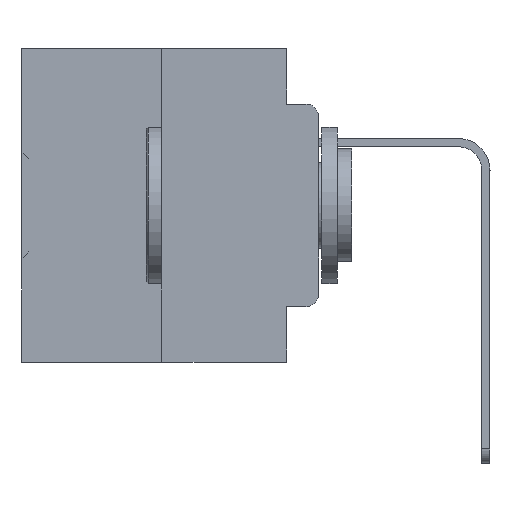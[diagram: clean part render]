
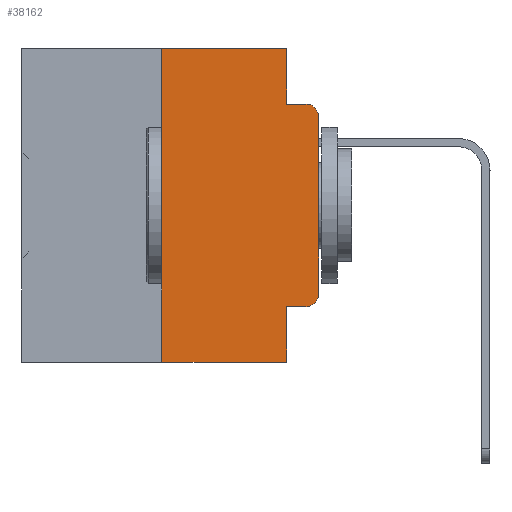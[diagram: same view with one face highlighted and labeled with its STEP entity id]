
A CAD part, left-side view. The second image highlights one B-rep face of the part: STEP entity #38162.
In plain terms, the highlighted planar face has unit normal (-1, 0, 0).
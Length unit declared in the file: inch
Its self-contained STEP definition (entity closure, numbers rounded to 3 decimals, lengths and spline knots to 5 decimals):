
#344 = DIRECTION ( 'NONE',  ( 0., -1., 0. ) ) ;
#496 = CARTESIAN_POINT ( 'NONE',  ( 0., 0.25, -0.5 ) ) ;
#507 = VECTOR ( 'NONE', #17823, 39.37008 ) ;
#673 = CARTESIAN_POINT ( 'NONE',  ( 0., 0.051, 0. ) ) ;
#3181 = VERTEX_POINT ( 'NONE', #29579 ) ;
#3183 = VERTEX_POINT ( 'NONE', #11912 ) ;
#3222 = CARTESIAN_POINT ( 'NONE',  ( 0., 0.473, -0.5 ) ) ;
#3623 = VERTEX_POINT ( 'NONE', #23403 ) ;
#4198 = ORIENTED_EDGE ( 'NONE', *, *, #27834, .T. ) ;
#4359 = LINE ( 'NONE', #6867, #10479 ) ;
#4739 = CARTESIAN_POINT ( 'NONE',  ( 0., 0.25, 0. ) ) ;
#5105 = ORIENTED_EDGE ( 'NONE', *, *, #22924, .T. ) ;
#5196 = FACE_OUTER_BOUND ( 'NONE', #33739, .T. ) ;
#6677 = AXIS2_PLACEMENT_3D ( 'NONE', #27060, #35985, #32703 ) ;
#6692 = EDGE_CURVE ( 'NONE', #25828, #33305, #9351, .T. ) ;
#6867 = CARTESIAN_POINT ( 'NONE',  ( 0., 0.473, 0. ) ) ;
#7886 = ORIENTED_EDGE ( 'NONE', *, *, #18816, .F. ) ;
#8548 = VECTOR ( 'NONE', #34842, 39.37008 ) ;
#9351 = LINE ( 'NONE', #18207, #34954 ) ;
#10479 = VECTOR ( 'NONE', #18948, 39.37008 ) ;
#10750 = EDGE_CURVE ( 'NONE', #22119, #18184, #4359, .T. ) ;
#11199 = ORIENTED_EDGE ( 'NONE', *, *, #17711, .F. ) ;
#11912 = CARTESIAN_POINT ( 'NONE',  ( 0., 0.051, -0.5 ) ) ;
#12039 = AXIS2_PLACEMENT_3D ( 'NONE', #25235, #18634, #13546 ) ;
#13354 = EDGE_CURVE ( 'NONE', #18184, #19110, #32192, .T. ) ;
#13495 = DIRECTION ( 'NONE',  ( 0., -1., 0. ) ) ;
#13541 = CARTESIAN_POINT ( 'NONE',  ( 0., 0.02, -0.3915 ) ) ;
#13546 = DIRECTION ( 'NONE',  ( 0., 0., -1. ) ) ;
#16390 = VECTOR ( 'NONE', #13495, 39.37008 ) ;
#17711 = EDGE_CURVE ( 'NONE', #35717, #22119, #23434, .T. ) ;
#17823 = DIRECTION ( 'NONE',  ( 0., -1., 0. ) ) ;
#18184 = VERTEX_POINT ( 'NONE', #673 ) ;
#18207 = CARTESIAN_POINT ( 'NONE',  ( 0., 0.051, -0.4115 ) ) ;
#18286 = LINE ( 'NONE', #34178, #16390 ) ;
#18634 = DIRECTION ( 'NONE',  ( -1., 0., 0. ) ) ;
#18816 = EDGE_CURVE ( 'NONE', #19110, #3181, #18286, .T. ) ;
#18948 = DIRECTION ( 'NONE',  ( 0., -1., 0. ) ) ;
#19110 = VERTEX_POINT ( 'NONE', #22458 ) ;
#19937 = ORIENTED_EDGE ( 'NONE', *, *, #6692, .T. ) ;
#20440 = LINE ( 'NONE', #25420, #37202 ) ;
#21006 = EDGE_CURVE ( 'NONE', #25828, #3183, #20440, .T. ) ;
#21831 = CARTESIAN_POINT ( 'NONE',  ( 0., 0.051, -0.4115 ) ) ;
#22119 = VERTEX_POINT ( 'NONE', #35613 ) ;
#22409 = ORIENTED_EDGE ( 'NONE', *, *, #34495, .T. ) ;
#22458 = CARTESIAN_POINT ( 'NONE',  ( 0., 0.051, -0.0885 ) ) ;
#22924 = EDGE_CURVE ( 'NONE', #35196, #3181, #33763, .T. ) ;
#23353 = VECTOR ( 'NONE', #23436, 39.37008 ) ;
#23403 = CARTESIAN_POINT ( 'NONE',  ( 0., 0., -0.3915 ) ) ;
#23434 = LINE ( 'NONE', #4739, #8548 ) ;
#23436 = DIRECTION ( 'NONE',  ( 0., 0., -1. ) ) ;
#24564 = CARTESIAN_POINT ( 'NONE',  ( 0., 0., 0. ) ) ;
#24969 = DIRECTION ( 'NONE',  ( 0., 0., -1. ) ) ;
#25235 = CARTESIAN_POINT ( 'NONE',  ( 0., 0.02, -0.1085 ) ) ;
#25420 = CARTESIAN_POINT ( 'NONE',  ( 0., 0.051, 0. ) ) ;
#25480 = DIRECTION ( 'NONE',  ( -1., 0., 0. ) ) ;
#25828 = VERTEX_POINT ( 'NONE', #21831 ) ;
#26255 = CARTESIAN_POINT ( 'NONE',  ( 0., 0.051, 0. ) ) ;
#26383 = VECTOR ( 'NONE', #36423, 39.37008 ) ;
#26831 = ORIENTED_EDGE ( 'NONE', *, *, #31840, .T. ) ;
#27060 = CARTESIAN_POINT ( 'NONE',  ( 0., 0.473, 0. ) ) ;
#27834 = EDGE_CURVE ( 'NONE', #35717, #3183, #28897, .T. ) ;
#28135 = DIRECTION ( 'NONE',  ( 0., 0., -1. ) ) ;
#28897 = LINE ( 'NONE', #3222, #507 ) ;
#29579 = CARTESIAN_POINT ( 'NONE',  ( 0., 0.02, -0.0885 ) ) ;
#30126 = CIRCLE ( 'NONE', #32931, 0.02 ) ;
#31840 = EDGE_CURVE ( 'NONE', #33305, #3623, #30126, .T. ) ;
#32192 = LINE ( 'NONE', #26255, #23353 ) ;
#32464 = ORIENTED_EDGE ( 'NONE', *, *, #21006, .F. ) ;
#32703 = DIRECTION ( 'NONE',  ( 0., 0., -1. ) ) ;
#32931 = AXIS2_PLACEMENT_3D ( 'NONE', #13541, #25480, #24969 ) ;
#32977 = PLANE ( 'NONE',  #6677 ) ;
#33305 = VERTEX_POINT ( 'NONE', #38333 ) ;
#33739 = EDGE_LOOP ( 'NONE', ( #22409, #5105, #7886, #35992, #37034, #11199, #4198, #32464, #19937, #26831 ) ) ;
#33763 = CIRCLE ( 'NONE', #12039, 0.02 ) ;
#34178 = CARTESIAN_POINT ( 'NONE',  ( 0., 0.051, -0.0885 ) ) ;
#34495 = EDGE_CURVE ( 'NONE', #3623, #35196, #37617, .T. ) ;
#34842 = DIRECTION ( 'NONE',  ( 0., 0., 1. ) ) ;
#34954 = VECTOR ( 'NONE', #344, 39.37008 ) ;
#35196 = VERTEX_POINT ( 'NONE', #37018 ) ;
#35613 = CARTESIAN_POINT ( 'NONE',  ( 0., 0.25, 0. ) ) ;
#35717 = VERTEX_POINT ( 'NONE', #496 ) ;
#35985 = DIRECTION ( 'NONE',  ( 1., 0., 0. ) ) ;
#35992 = ORIENTED_EDGE ( 'NONE', *, *, #13354, .F. ) ;
#36423 = DIRECTION ( 'NONE',  ( 0., 0., 1. ) ) ;
#37018 = CARTESIAN_POINT ( 'NONE',  ( 0., 0., -0.1085 ) ) ;
#37034 = ORIENTED_EDGE ( 'NONE', *, *, #10750, .F. ) ;
#37202 = VECTOR ( 'NONE', #28135, 39.37008 ) ;
#37617 = LINE ( 'NONE', #24564, #26383 ) ;
#38162 = ADVANCED_FACE ( 'NONE', ( #5196 ), #32977, .F. ) ;
#38333 = CARTESIAN_POINT ( 'NONE',  ( 0., 0.02, -0.4115 ) ) ;
